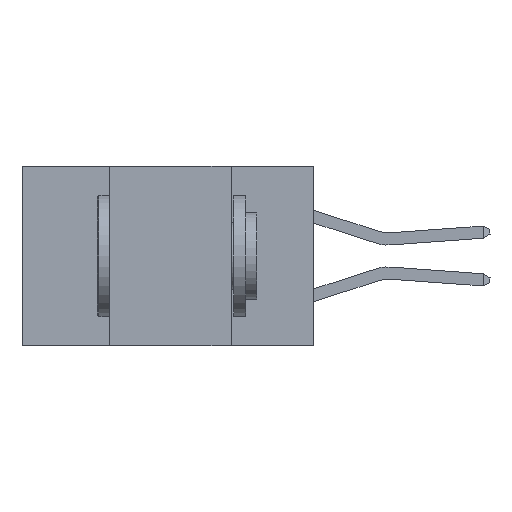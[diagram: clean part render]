
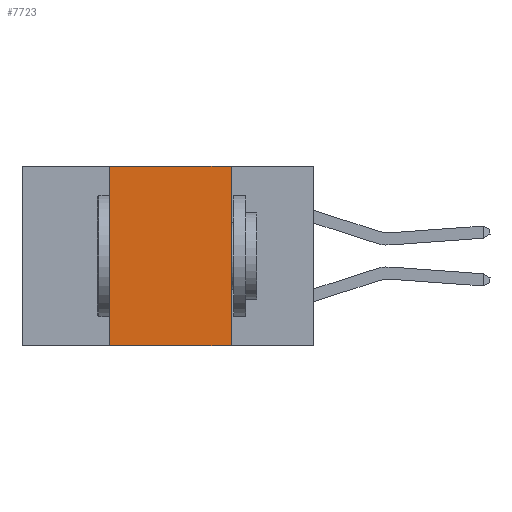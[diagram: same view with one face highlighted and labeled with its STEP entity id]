
A CAD part, left-side view. The second image highlights one B-rep face of the part: STEP entity #7723.
In plain terms, the highlighted planar face has unit normal (-1, 0, 0).
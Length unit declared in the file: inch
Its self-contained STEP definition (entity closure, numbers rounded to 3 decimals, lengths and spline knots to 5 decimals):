
#952 = ORIENTED_EDGE ( 'NONE', *, *, #3617, .F. ) ;
#2140 = ORIENTED_EDGE ( 'NONE', *, *, #17777, .F. ) ;
#2707 = VECTOR ( 'NONE', #27760, 39.37008 ) ;
#3617 = EDGE_CURVE ( 'NONE', #17083, #22603, #17227, .T. ) ;
#3618 = DIRECTION ( 'NONE',  ( 0., 0., -1. ) ) ;
#5477 = CARTESIAN_POINT ( 'NONE',  ( 0., 0.6, -0.37 ) ) ;
#5672 = DIRECTION ( 'NONE',  ( 0., -1., 0. ) ) ;
#5977 = LINE ( 'NONE', #5477, #21737 ) ;
#6315 = EDGE_CURVE ( 'NONE', #22805, #22603, #5977, .T. ) ;
#6988 = AXIS2_PLACEMENT_3D ( 'NONE', #15914, #26257, #3618 ) ;
#7427 = CARTESIAN_POINT ( 'NONE',  ( 0., 0.42, 0. ) ) ;
#7723 = ADVANCED_FACE ( 'NONE', ( #30372 ), #23270, .F. ) ;
#9758 = VECTOR ( 'NONE', #10401, 39.37008 ) ;
#10087 = ORIENTED_EDGE ( 'NONE', *, *, #29813, .F. ) ;
#10401 = DIRECTION ( 'NONE',  ( 0., 0., -1. ) ) ;
#10951 = LINE ( 'NONE', #7427, #2707 ) ;
#12143 = EDGE_LOOP ( 'NONE', ( #952, #10087, #2140, #19592 ) ) ;
#15914 = CARTESIAN_POINT ( 'NONE',  ( 0., 0.6, 0. ) ) ;
#15980 = VECTOR ( 'NONE', #5672, 39.37008 ) ;
#17083 = VERTEX_POINT ( 'NONE', #18635 ) ;
#17227 = LINE ( 'NONE', #22599, #9758 ) ;
#17777 = EDGE_CURVE ( 'NONE', #22805, #20441, #10951, .T. ) ;
#18635 = CARTESIAN_POINT ( 'NONE',  ( 0., 0.17, 0. ) ) ;
#19592 = ORIENTED_EDGE ( 'NONE', *, *, #6315, .T. ) ;
#20441 = VERTEX_POINT ( 'NONE', #28119 ) ;
#20728 = CARTESIAN_POINT ( 'NONE',  ( 0., 0.6, 0. ) ) ;
#21078 = LINE ( 'NONE', #20728, #15980 ) ;
#21737 = VECTOR ( 'NONE', #27928, 39.37008 ) ;
#22599 = CARTESIAN_POINT ( 'NONE',  ( 0., 0.17, 0. ) ) ;
#22603 = VERTEX_POINT ( 'NONE', #22730 ) ;
#22730 = CARTESIAN_POINT ( 'NONE',  ( 0., 0.17, -0.37 ) ) ;
#22805 = VERTEX_POINT ( 'NONE', #22929 ) ;
#22929 = CARTESIAN_POINT ( 'NONE',  ( 0., 0.42, -0.37 ) ) ;
#23270 = PLANE ( 'NONE',  #6988 ) ;
#26257 = DIRECTION ( 'NONE',  ( 1., 0., 0. ) ) ;
#27760 = DIRECTION ( 'NONE',  ( 0., 0., 1. ) ) ;
#27928 = DIRECTION ( 'NONE',  ( 0., -1., 0. ) ) ;
#28119 = CARTESIAN_POINT ( 'NONE',  ( 0., 0.42, 0. ) ) ;
#29813 = EDGE_CURVE ( 'NONE', #20441, #17083, #21078, .T. ) ;
#30372 = FACE_OUTER_BOUND ( 'NONE', #12143, .T. ) ;
